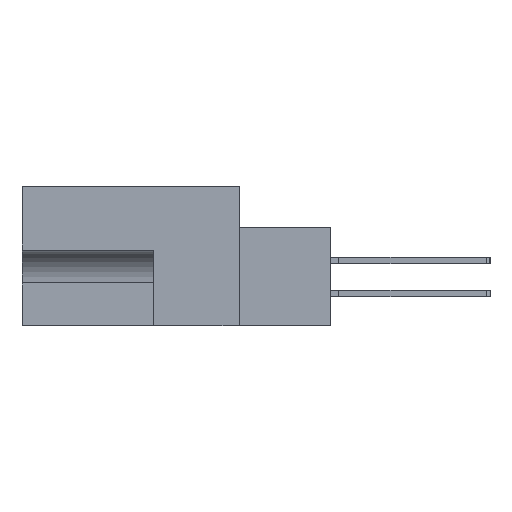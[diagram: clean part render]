
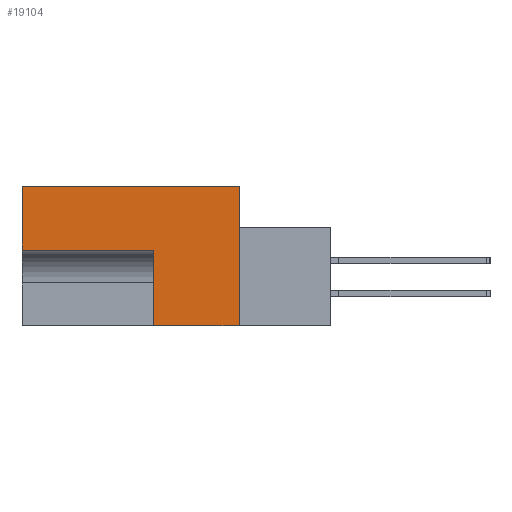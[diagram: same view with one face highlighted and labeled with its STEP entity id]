
A CAD part, left-side view. The second image highlights one B-rep face of the part: STEP entity #19104.
In plain terms, the highlighted planar face has unit normal (-1, 0, 0).
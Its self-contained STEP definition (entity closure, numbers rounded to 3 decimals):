
#849 = LINE ( 'NONE', #24378, #2549 ) ;
#939 = LINE ( 'NONE', #3040, #24810 ) ;
#2549 = VECTOR ( 'NONE', #18799, 1000. ) ;
#2621 = DIRECTION ( 'NONE',  ( 0., 0., -1. ) ) ;
#2674 = EDGE_CURVE ( 'NONE', #11115, #27771, #3984, .T. ) ;
#3040 = CARTESIAN_POINT ( 'NONE',  ( 0., -8.814, -13.487 ) ) ;
#3714 = VERTEX_POINT ( 'NONE', #18540 ) ;
#3984 = LINE ( 'NONE', #9427, #32088 ) ;
#5181 = VERTEX_POINT ( 'NONE', #34685 ) ;
#5377 = DIRECTION ( 'NONE',  ( 1., 0., 0. ) ) ;
#6546 = LINE ( 'NONE', #18355, #13343 ) ;
#8281 = CARTESIAN_POINT ( 'NONE',  ( 0., 11.506, 0. ) ) ;
#8445 = CARTESIAN_POINT ( 'NONE',  ( 0., 0., 0. ) ) ;
#9062 = ORIENTED_EDGE ( 'NONE', *, *, #11358, .F. ) ;
#9427 = CARTESIAN_POINT ( 'NONE',  ( 0., 20.955, -13.487 ) ) ;
#9848 = EDGE_CURVE ( 'NONE', #5181, #22079, #939, .T. ) ;
#11115 = VERTEX_POINT ( 'NONE', #34617 ) ;
#11358 = EDGE_CURVE ( 'NONE', #3714, #11115, #849, .T. ) ;
#12024 = LINE ( 'NONE', #8281, #17578 ) ;
#12275 = LINE ( 'NONE', #31542, #33997 ) ;
#13343 = VECTOR ( 'NONE', #15719, 1000. ) ;
#15195 = ORIENTED_EDGE ( 'NONE', *, *, #2674, .F. ) ;
#15261 = VERTEX_POINT ( 'NONE', #29951 ) ;
#15719 = DIRECTION ( 'NONE',  ( 0., 0., -1. ) ) ;
#16236 = ORIENTED_EDGE ( 'NONE', *, *, #9848, .F. ) ;
#17578 = VECTOR ( 'NONE', #32958, 1000. ) ;
#18355 = CARTESIAN_POINT ( 'NONE',  ( 0., 0., 0. ) ) ;
#18540 = CARTESIAN_POINT ( 'NONE',  ( 0., 8.255, -6.172 ) ) ;
#18799 = DIRECTION ( 'NONE',  ( 0., 1., 0. ) ) ;
#19104 = ADVANCED_FACE ( 'NONE', ( #24716 ), #32892, .F. ) ;
#19318 = ORIENTED_EDGE ( 'NONE', *, *, #28896, .F. ) ;
#22079 = VERTEX_POINT ( 'NONE', #28033 ) ;
#22335 = CARTESIAN_POINT ( 'NONE',  ( 0., 20.955, 0. ) ) ;
#22581 = DIRECTION ( 'NONE',  ( 0., 0., 1. ) ) ;
#23188 = EDGE_LOOP ( 'NONE', ( #16236, #19318, #27832, #15195, #9062, #33887 ) ) ;
#24378 = CARTESIAN_POINT ( 'NONE',  ( 0., 8.255, -6.172 ) ) ;
#24716 = FACE_OUTER_BOUND ( 'NONE', #23188, .T. ) ;
#24810 = VECTOR ( 'NONE', #30181, 1000. ) ;
#25576 = EDGE_CURVE ( 'NONE', #27771, #15261, #12024, .T. ) ;
#27771 = VERTEX_POINT ( 'NONE', #22335 ) ;
#27832 = ORIENTED_EDGE ( 'NONE', *, *, #25576, .F. ) ;
#28033 = CARTESIAN_POINT ( 'NONE',  ( 0., 8.255, -13.487 ) ) ;
#28402 = AXIS2_PLACEMENT_3D ( 'NONE', #8445, #5377, #2621 ) ;
#28896 = EDGE_CURVE ( 'NONE', #15261, #5181, #6546, .T. ) ;
#29951 = CARTESIAN_POINT ( 'NONE',  ( 0., 0., 0. ) ) ;
#30181 = DIRECTION ( 'NONE',  ( 0., 1., 0. ) ) ;
#31542 = CARTESIAN_POINT ( 'NONE',  ( 0., 8.255, -13.487 ) ) ;
#31656 = DIRECTION ( 'NONE',  ( 0., 0., 1. ) ) ;
#31802 = EDGE_CURVE ( 'NONE', #22079, #3714, #12275, .T. ) ;
#32088 = VECTOR ( 'NONE', #22581, 1000. ) ;
#32892 = PLANE ( 'NONE',  #28402 ) ;
#32958 = DIRECTION ( 'NONE',  ( 0., -1., 0. ) ) ;
#33887 = ORIENTED_EDGE ( 'NONE', *, *, #31802, .F. ) ;
#33997 = VECTOR ( 'NONE', #31656, 1000. ) ;
#34617 = CARTESIAN_POINT ( 'NONE',  ( 0., 20.955, -6.172 ) ) ;
#34685 = CARTESIAN_POINT ( 'NONE',  ( 0., 0., -13.487 ) ) ;
